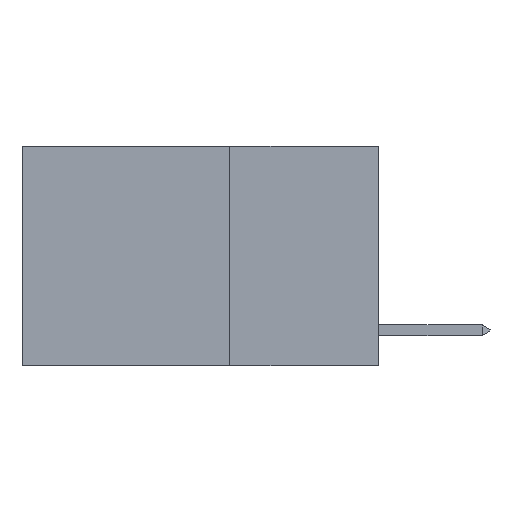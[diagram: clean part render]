
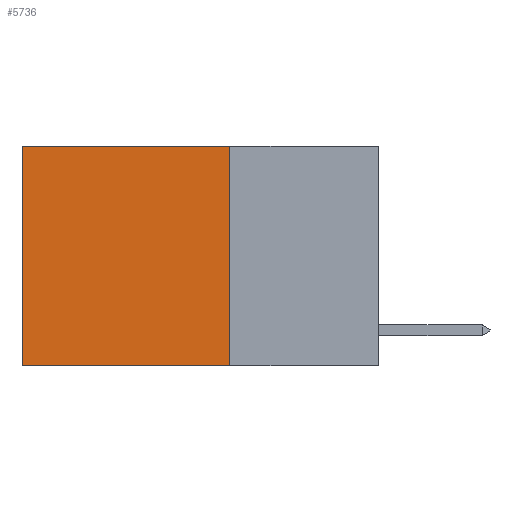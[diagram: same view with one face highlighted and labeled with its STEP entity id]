
A CAD part, left-side view. The second image highlights one B-rep face of the part: STEP entity #5736.
In plain terms, the highlighted planar face has unit normal (-1, 0, 0).
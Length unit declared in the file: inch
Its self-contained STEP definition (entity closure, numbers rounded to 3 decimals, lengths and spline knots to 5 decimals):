
#155 = CARTESIAN_POINT ( 'NONE',  ( 0.2625, 0.6, 0. ) ) ;
#322 = VERTEX_POINT ( 'NONE', #10293 ) ;
#978 = AXIS2_PLACEMENT_3D ( 'NONE', #5371, #19063, #21005 ) ;
#1006 = LINE ( 'NONE', #25777, #5336 ) ;
#1422 = LINE ( 'NONE', #10594, #27284 ) ;
#2570 = ORIENTED_EDGE ( 'NONE', *, *, #14432, .T. ) ;
#3828 = EDGE_CURVE ( 'NONE', #26829, #322, #1422, .T. ) ;
#5279 = VECTOR ( 'NONE', #16086, 39.37008 ) ;
#5336 = VECTOR ( 'NONE', #12345, 39.37008 ) ;
#5371 = CARTESIAN_POINT ( 'NONE',  ( 0.2625, 0.25, 0. ) ) ;
#5736 = ADVANCED_FACE ( 'NONE', ( #25558 ), #25284, .F. ) ;
#6265 = CARTESIAN_POINT ( 'NONE',  ( 0.2625, 0.6, -0.37 ) ) ;
#7681 = VECTOR ( 'NONE', #11326, 39.37008 ) ;
#10293 = CARTESIAN_POINT ( 'NONE',  ( 0.2625, 0.25, -0.37 ) ) ;
#10594 = CARTESIAN_POINT ( 'NONE',  ( 0.2625, 0.25, 0. ) ) ;
#11326 = DIRECTION ( 'NONE',  ( 0., 1., 0. ) ) ;
#12345 = DIRECTION ( 'NONE',  ( 0., 1., 0. ) ) ;
#14432 = EDGE_CURVE ( 'NONE', #26829, #28573, #20484, .T. ) ;
#15526 = CARTESIAN_POINT ( 'NONE',  ( 0.2625, 0.6, 0. ) ) ;
#16086 = DIRECTION ( 'NONE',  ( 0., 0., -1. ) ) ;
#18355 = ORIENTED_EDGE ( 'NONE', *, *, #27648, .F. ) ;
#19063 = DIRECTION ( 'NONE',  ( 1., 0., 0. ) ) ;
#19123 = DIRECTION ( 'NONE',  ( 0., 0., -1. ) ) ;
#19896 = CARTESIAN_POINT ( 'NONE',  ( 0.2625, 0.25, 0. ) ) ;
#19992 = CARTESIAN_POINT ( 'NONE',  ( 0.2625, 0.25, 0. ) ) ;
#20484 = LINE ( 'NONE', #19896, #7681 ) ;
#21005 = DIRECTION ( 'NONE',  ( 0., 0., -1. ) ) ;
#21530 = EDGE_LOOP ( 'NONE', ( #26164, #18355, #27718, #2570 ) ) ;
#24305 = VERTEX_POINT ( 'NONE', #6265 ) ;
#24653 = LINE ( 'NONE', #155, #5279 ) ;
#25284 = PLANE ( 'NONE',  #978 ) ;
#25558 = FACE_OUTER_BOUND ( 'NONE', #21530, .T. ) ;
#25777 = CARTESIAN_POINT ( 'NONE',  ( 0.2625, 0.25, -0.37 ) ) ;
#26056 = EDGE_CURVE ( 'NONE', #28573, #24305, #24653, .T. ) ;
#26164 = ORIENTED_EDGE ( 'NONE', *, *, #26056, .T. ) ;
#26829 = VERTEX_POINT ( 'NONE', #19992 ) ;
#27284 = VECTOR ( 'NONE', #19123, 39.37008 ) ;
#27648 = EDGE_CURVE ( 'NONE', #322, #24305, #1006, .T. ) ;
#27718 = ORIENTED_EDGE ( 'NONE', *, *, #3828, .F. ) ;
#28573 = VERTEX_POINT ( 'NONE', #15526 ) ;
